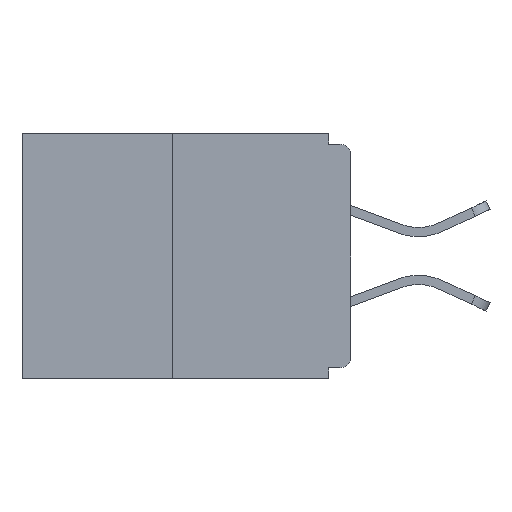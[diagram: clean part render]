
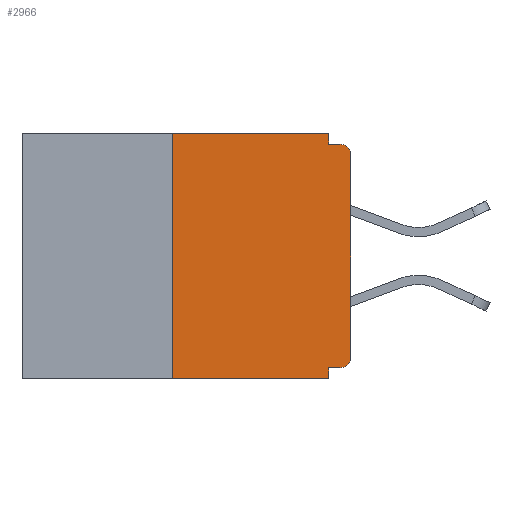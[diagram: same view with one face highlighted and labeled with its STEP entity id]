
A CAD part, left-side view. The second image highlights one B-rep face of the part: STEP entity #2966.
In plain terms, the highlighted planar face has unit normal (-1, 0, 0).
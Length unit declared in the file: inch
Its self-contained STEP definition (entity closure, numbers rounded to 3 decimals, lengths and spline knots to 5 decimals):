
#145 = VERTEX_POINT ( 'NONE', #1811 ) ;
#226 = VECTOR ( 'NONE', #29521, 39.37008 ) ;
#261 = EDGE_CURVE ( 'NONE', #2135, #23769, #529, .T. ) ;
#529 = LINE ( 'NONE', #29257, #8032 ) ;
#560 = DIRECTION ( 'NONE',  ( 0., -1., 0. ) ) ;
#729 = EDGE_CURVE ( 'NONE', #24036, #21406, #4055, .T. ) ;
#1144 = VECTOR ( 'NONE', #9641, 39.37008 ) ;
#1216 = PLANE ( 'NONE',  #12274 ) ;
#1811 = CARTESIAN_POINT ( 'NONE',  ( 0., 0.25, 0. ) ) ;
#1871 = DIRECTION ( 'NONE',  ( 0., -1., 0. ) ) ;
#1899 = EDGE_CURVE ( 'NONE', #14082, #24036, #12193, .T. ) ;
#1915 = EDGE_CURVE ( 'NONE', #13505, #6631, #16479, .T. ) ;
#2135 = VERTEX_POINT ( 'NONE', #25759 ) ;
#2696 = DIRECTION ( 'NONE',  ( 0., 1., 0. ) ) ;
#2826 = ORIENTED_EDGE ( 'NONE', *, *, #19643, .T. ) ;
#2960 = CARTESIAN_POINT ( 'NONE',  ( 0., 0.031, -0.015 ) ) ;
#2966 = ADVANCED_FACE ( 'NONE', ( #23607 ), #1216, .F. ) ;
#4001 = LINE ( 'NONE', #9043, #1144 ) ;
#4055 = LINE ( 'NONE', #6259, #12958 ) ;
#4282 = CARTESIAN_POINT ( 'NONE',  ( 0., 0.015, -0.328 ) ) ;
#4415 = AXIS2_PLACEMENT_3D ( 'NONE', #21967, #19762, #5984 ) ;
#4609 = CARTESIAN_POINT ( 'NONE',  ( 0., 0.25, -0.343 ) ) ;
#4829 = LINE ( 'NONE', #23271, #22336 ) ;
#5606 = CARTESIAN_POINT ( 'NONE',  ( 0., 0.46, 0. ) ) ;
#5984 = DIRECTION ( 'NONE',  ( 0., 0., -1. ) ) ;
#6259 = CARTESIAN_POINT ( 'NONE',  ( 0., 0., -0.015 ) ) ;
#6631 = VERTEX_POINT ( 'NONE', #18339 ) ;
#7030 = VERTEX_POINT ( 'NONE', #22433 ) ;
#7148 = EDGE_CURVE ( 'NONE', #24929, #145, #7729, .T. ) ;
#7431 = EDGE_CURVE ( 'NONE', #145, #14082, #18418, .T. ) ;
#7729 = LINE ( 'NONE', #22832, #226 ) ;
#7793 = VECTOR ( 'NONE', #560, 39.37008 ) ;
#8032 = VECTOR ( 'NONE', #24763, 39.37008 ) ;
#8086 = DIRECTION ( 'NONE',  ( 1., 0., 0. ) ) ;
#9043 = CARTESIAN_POINT ( 'NONE',  ( 0., 0., 0. ) ) ;
#9641 = DIRECTION ( 'NONE',  ( 0., 0., 1. ) ) ;
#10054 = ORIENTED_EDGE ( 'NONE', *, *, #17914, .F. ) ;
#10216 = ORIENTED_EDGE ( 'NONE', *, *, #7148, .F. ) ;
#10237 = EDGE_LOOP ( 'NONE', ( #27209, #10216, #16385, #24126, #10054, #10902, #2826, #21951, #12135, #26014 ) ) ;
#10382 = DIRECTION ( 'NONE',  ( 0., 0., -1. ) ) ;
#10902 = ORIENTED_EDGE ( 'NONE', *, *, #1915, .T. ) ;
#11219 = EDGE_CURVE ( 'NONE', #7030, #21406, #28214, .T. ) ;
#11673 = LINE ( 'NONE', #11908, #7793 ) ;
#11908 = CARTESIAN_POINT ( 'NONE',  ( 0., 0.46, -0.343 ) ) ;
#12135 = ORIENTED_EDGE ( 'NONE', *, *, #729, .F. ) ;
#12193 = LINE ( 'NONE', #24676, #16124 ) ;
#12274 = AXIS2_PLACEMENT_3D ( 'NONE', #5606, #8086, #10382 ) ;
#12958 = VECTOR ( 'NONE', #1871, 39.37008 ) ;
#13262 = DIRECTION ( 'NONE',  ( -1., 0., 0. ) ) ;
#13505 = VERTEX_POINT ( 'NONE', #4282 ) ;
#14082 = VERTEX_POINT ( 'NONE', #23110 ) ;
#16124 = VECTOR ( 'NONE', #17770, 39.37008 ) ;
#16385 = ORIENTED_EDGE ( 'NONE', *, *, #26285, .T. ) ;
#16479 = CIRCLE ( 'NONE', #28925, 0.015 ) ;
#17544 = CARTESIAN_POINT ( 'NONE',  ( 0., 0.015, -0.015 ) ) ;
#17770 = DIRECTION ( 'NONE',  ( 0., 0., -1. ) ) ;
#17914 = EDGE_CURVE ( 'NONE', #13505, #2135, #4829, .T. ) ;
#18339 = CARTESIAN_POINT ( 'NONE',  ( 0., 0., -0.313 ) ) ;
#18418 = LINE ( 'NONE', #21546, #29133 ) ;
#19643 = EDGE_CURVE ( 'NONE', #6631, #7030, #4001, .T. ) ;
#19762 = DIRECTION ( 'NONE',  ( -1., 0., 0. ) ) ;
#21406 = VERTEX_POINT ( 'NONE', #17544 ) ;
#21546 = CARTESIAN_POINT ( 'NONE',  ( 0., 0.46, 0. ) ) ;
#21951 = ORIENTED_EDGE ( 'NONE', *, *, #11219, .T. ) ;
#21967 = CARTESIAN_POINT ( 'NONE',  ( 0., 0.015, -0.03 ) ) ;
#22336 = VECTOR ( 'NONE', #2696, 39.37008 ) ;
#22433 = CARTESIAN_POINT ( 'NONE',  ( 0., 0., -0.03 ) ) ;
#22832 = CARTESIAN_POINT ( 'NONE',  ( 0., 0.25, 0. ) ) ;
#23110 = CARTESIAN_POINT ( 'NONE',  ( 0., 0.031, 0. ) ) ;
#23271 = CARTESIAN_POINT ( 'NONE',  ( 0., 0., -0.328 ) ) ;
#23607 = FACE_OUTER_BOUND ( 'NONE', #10237, .T. ) ;
#23769 = VERTEX_POINT ( 'NONE', #26729 ) ;
#24036 = VERTEX_POINT ( 'NONE', #2960 ) ;
#24126 = ORIENTED_EDGE ( 'NONE', *, *, #261, .F. ) ;
#24676 = CARTESIAN_POINT ( 'NONE',  ( 0., 0.031, 0. ) ) ;
#24763 = DIRECTION ( 'NONE',  ( 0., 0., -1. ) ) ;
#24929 = VERTEX_POINT ( 'NONE', #4609 ) ;
#25759 = CARTESIAN_POINT ( 'NONE',  ( 0., 0.031, -0.328 ) ) ;
#25999 = DIRECTION ( 'NONE',  ( 0., -1., 0. ) ) ;
#26014 = ORIENTED_EDGE ( 'NONE', *, *, #1899, .F. ) ;
#26285 = EDGE_CURVE ( 'NONE', #24929, #23769, #11673, .T. ) ;
#26660 = DIRECTION ( 'NONE',  ( 0., 0., -1. ) ) ;
#26729 = CARTESIAN_POINT ( 'NONE',  ( 0., 0.031, -0.343 ) ) ;
#27209 = ORIENTED_EDGE ( 'NONE', *, *, #7431, .F. ) ;
#28214 = CIRCLE ( 'NONE', #4415, 0.015 ) ;
#28925 = AXIS2_PLACEMENT_3D ( 'NONE', #29166, #13262, #26660 ) ;
#29133 = VECTOR ( 'NONE', #25999, 39.37008 ) ;
#29166 = CARTESIAN_POINT ( 'NONE',  ( 0., 0.015, -0.313 ) ) ;
#29257 = CARTESIAN_POINT ( 'NONE',  ( 0., 0.031, -0.343 ) ) ;
#29521 = DIRECTION ( 'NONE',  ( 0., 0., 1. ) ) ;
